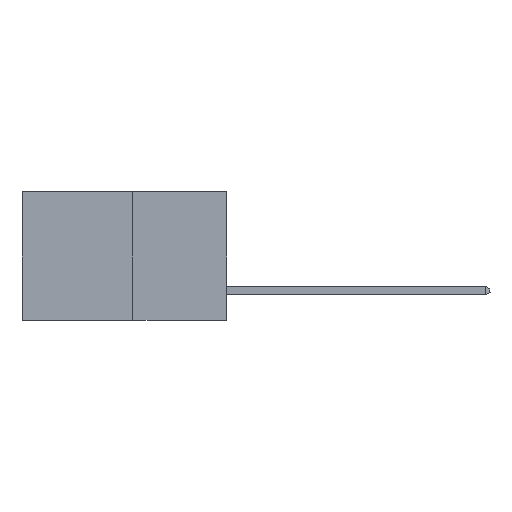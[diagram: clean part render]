
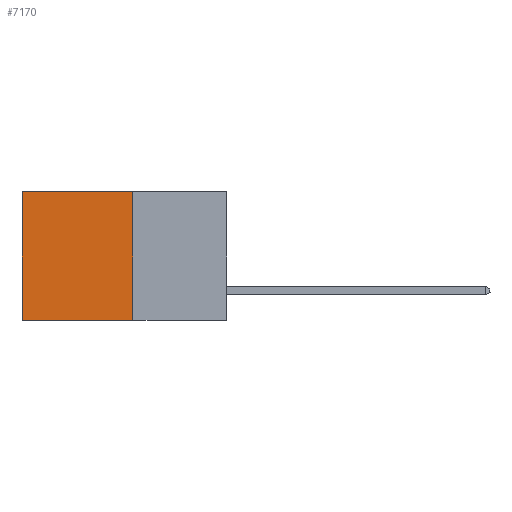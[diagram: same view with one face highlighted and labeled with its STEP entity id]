
A CAD part, left-side view. The second image highlights one B-rep face of the part: STEP entity #7170.
In plain terms, the highlighted planar face has unit normal (-1, 0, 0).
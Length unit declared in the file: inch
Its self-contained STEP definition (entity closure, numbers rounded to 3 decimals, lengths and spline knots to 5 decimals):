
#133 = CARTESIAN_POINT ( 'NONE',  ( 0.277, 0.59, 0. ) ) ;
#154 = LINE ( 'NONE', #17291, #22907 ) ;
#844 = CARTESIAN_POINT ( 'NONE',  ( 0.277, 0.27, -0.37 ) ) ;
#984 = VECTOR ( 'NONE', #13077, 39.37008 ) ;
#1560 = EDGE_CURVE ( 'NONE', #13828, #27832, #6925, .T. ) ;
#1719 = DIRECTION ( 'NONE',  ( 0., 0., -1. ) ) ;
#4666 = AXIS2_PLACEMENT_3D ( 'NONE', #10118, #18951, #5677 ) ;
#5677 = DIRECTION ( 'NONE',  ( 0., 0., -1. ) ) ;
#6142 = CARTESIAN_POINT ( 'NONE',  ( 0.277, 0.59, -0.37 ) ) ;
#6925 = LINE ( 'NONE', #13172, #984 ) ;
#7170 = ADVANCED_FACE ( 'NONE', ( #14325 ), #25361, .F. ) ;
#7478 = DIRECTION ( 'NONE',  ( 0., 0., -1. ) ) ;
#7506 = CARTESIAN_POINT ( 'NONE',  ( 0.277, 0.27, 0. ) ) ;
#9372 = LINE ( 'NONE', #7506, #20348 ) ;
#9429 = VERTEX_POINT ( 'NONE', #133 ) ;
#9475 = ORIENTED_EDGE ( 'NONE', *, *, #19453, .T. ) ;
#9660 = CARTESIAN_POINT ( 'NONE',  ( 0.277, 0.27, -0.37 ) ) ;
#10118 = CARTESIAN_POINT ( 'NONE',  ( 0.277, 0.27, -0.37 ) ) ;
#11048 = EDGE_CURVE ( 'NONE', #21909, #13828, #17077, .T. ) ;
#13077 = DIRECTION ( 'NONE',  ( 0., 1., 0. ) ) ;
#13172 = CARTESIAN_POINT ( 'NONE',  ( 0.277, 0.27, -0.37 ) ) ;
#13828 = VERTEX_POINT ( 'NONE', #9660 ) ;
#14325 = FACE_OUTER_BOUND ( 'NONE', #20858, .T. ) ;
#14426 = ORIENTED_EDGE ( 'NONE', *, *, #17412, .T. ) ;
#15939 = ORIENTED_EDGE ( 'NONE', *, *, #1560, .F. ) ;
#16482 = DIRECTION ( 'NONE',  ( 0., 1., 0. ) ) ;
#17077 = LINE ( 'NONE', #844, #22095 ) ;
#17291 = CARTESIAN_POINT ( 'NONE',  ( 0.277, 0.59, -0.37 ) ) ;
#17412 = EDGE_CURVE ( 'NONE', #21909, #9429, #9372, .T. ) ;
#18951 = DIRECTION ( 'NONE',  ( 1., 0., 0. ) ) ;
#19453 = EDGE_CURVE ( 'NONE', #9429, #27832, #154, .T. ) ;
#19990 = ORIENTED_EDGE ( 'NONE', *, *, #11048, .F. ) ;
#20348 = VECTOR ( 'NONE', #16482, 39.37008 ) ;
#20858 = EDGE_LOOP ( 'NONE', ( #9475, #15939, #19990, #14426 ) ) ;
#21909 = VERTEX_POINT ( 'NONE', #23360 ) ;
#22095 = VECTOR ( 'NONE', #7478, 39.37008 ) ;
#22907 = VECTOR ( 'NONE', #1719, 39.37008 ) ;
#23360 = CARTESIAN_POINT ( 'NONE',  ( 0.277, 0.27, 0. ) ) ;
#25361 = PLANE ( 'NONE',  #4666 ) ;
#27832 = VERTEX_POINT ( 'NONE', #6142 ) ;
